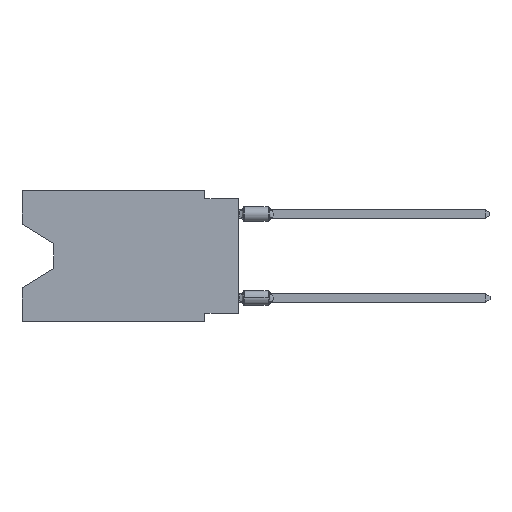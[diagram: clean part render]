
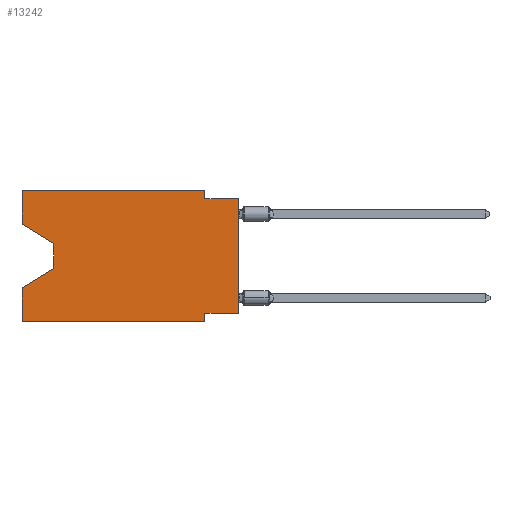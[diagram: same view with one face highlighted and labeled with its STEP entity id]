
A CAD part, left-side view. The second image highlights one B-rep face of the part: STEP entity #13242.
In plain terms, the highlighted planar face has unit normal (-1, 0, 0).
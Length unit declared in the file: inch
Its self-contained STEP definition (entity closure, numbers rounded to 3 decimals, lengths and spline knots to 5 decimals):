
#98 = DIRECTION ( 'NONE',  ( 1., 0., 0. ) ) ;
#227 = VERTEX_POINT ( 'NONE', #9976 ) ;
#761 = VERTEX_POINT ( 'NONE', #15942 ) ;
#2110 = ORIENTED_EDGE ( 'NONE', *, *, #5034, .F. ) ;
#2157 = CARTESIAN_POINT ( 'NONE',  ( 0., 0.1, -0.025 ) ) ;
#2492 = VECTOR ( 'NONE', #20686, 39.37008 ) ;
#2521 = VERTEX_POINT ( 'NONE', #2764 ) ;
#2705 = ORIENTED_EDGE ( 'NONE', *, *, #11170, .F. ) ;
#2764 = CARTESIAN_POINT ( 'NONE',  ( 0., 0., -0.025 ) ) ;
#2971 = EDGE_CURVE ( 'NONE', #761, #23270, #11813, .T. ) ;
#3758 = EDGE_CURVE ( 'NONE', #20661, #7375, #24118, .T. ) ;
#3855 = LINE ( 'NONE', #13872, #32271 ) ;
#4370 = CARTESIAN_POINT ( 'NONE',  ( 0., 0.645, -0.39 ) ) ;
#4627 = VECTOR ( 'NONE', #27420, 39.37008 ) ;
#4654 = DIRECTION ( 'NONE',  ( 0., -1., 0. ) ) ;
#5034 = EDGE_CURVE ( 'NONE', #16988, #2521, #13392, .T. ) ;
#5116 = ORIENTED_EDGE ( 'NONE', *, *, #30022, .F. ) ;
#5453 = AXIS2_PLACEMENT_3D ( 'NONE', #20775, #98, #15460 ) ;
#5732 = ORIENTED_EDGE ( 'NONE', *, *, #14408, .F. ) ;
#5986 = DIRECTION ( 'NONE',  ( 0., -1., 0. ) ) ;
#6054 = DIRECTION ( 'NONE',  ( 0., -1., 0. ) ) ;
#6690 = DIRECTION ( 'NONE',  ( 0., 0., -1. ) ) ;
#7098 = CARTESIAN_POINT ( 'NONE',  ( 0., 0.645, 0. ) ) ;
#7127 = EDGE_CURVE ( 'NONE', #15170, #16988, #24816, .T. ) ;
#7375 = VERTEX_POINT ( 'NONE', #26472 ) ;
#8446 = VECTOR ( 'NONE', #6690, 39.37008 ) ;
#9306 = CARTESIAN_POINT ( 'NONE',  ( 0., 0.1, -0.39 ) ) ;
#9571 = CARTESIAN_POINT ( 'NONE',  ( 0., 0.645, -0.10025 ) ) ;
#9764 = EDGE_CURVE ( 'NONE', #227, #2521, #15605, .T. ) ;
#9976 = CARTESIAN_POINT ( 'NONE',  ( 0., 0., -0.365 ) ) ;
#10005 = LINE ( 'NONE', #12577, #27619 ) ;
#10210 = LINE ( 'NONE', #7098, #2492 ) ;
#10726 = VECTOR ( 'NONE', #30234, 39.37008 ) ;
#11064 = CARTESIAN_POINT ( 'NONE',  ( 0., 0.645, -0.39 ) ) ;
#11170 = EDGE_CURVE ( 'NONE', #227, #29761, #3855, .T. ) ;
#11813 = LINE ( 'NONE', #9571, #15430 ) ;
#11831 = ORIENTED_EDGE ( 'NONE', *, *, #21192, .T. ) ;
#11841 = CARTESIAN_POINT ( 'NONE',  ( 0., 0.55, -0.158 ) ) ;
#12103 = EDGE_CURVE ( 'NONE', #29761, #7375, #28031, .T. ) ;
#12191 = ORIENTED_EDGE ( 'NONE', *, *, #3758, .T. ) ;
#12577 = CARTESIAN_POINT ( 'NONE',  ( 0., 0.645, 0. ) ) ;
#12833 = ORIENTED_EDGE ( 'NONE', *, *, #7127, .F. ) ;
#13202 = FACE_OUTER_BOUND ( 'NONE', #30408, .T. ) ;
#13242 = ADVANCED_FACE ( 'NONE', ( #13202 ), #28349, .F. ) ;
#13392 = LINE ( 'NONE', #29064, #26580 ) ;
#13872 = CARTESIAN_POINT ( 'NONE',  ( 0., 0., -0.365 ) ) ;
#14408 = EDGE_CURVE ( 'NONE', #26489, #15170, #10005, .T. ) ;
#14810 = DIRECTION ( 'NONE',  ( 0., 0., -1. ) ) ;
#15029 = CARTESIAN_POINT ( 'NONE',  ( 0., 0.645, 0. ) ) ;
#15170 = VERTEX_POINT ( 'NONE', #26195 ) ;
#15373 = ORIENTED_EDGE ( 'NONE', *, *, #16788, .F. ) ;
#15430 = VECTOR ( 'NONE', #27621, 39.37008 ) ;
#15460 = DIRECTION ( 'NONE',  ( 0., 0., -1. ) ) ;
#15471 = VERTEX_POINT ( 'NONE', #27386 ) ;
#15605 = LINE ( 'NONE', #23324, #16844 ) ;
#15942 = CARTESIAN_POINT ( 'NONE',  ( 0., 0.645, -0.10025 ) ) ;
#16788 = EDGE_CURVE ( 'NONE', #761, #26489, #17499, .T. ) ;
#16844 = VECTOR ( 'NONE', #18684, 39.37008 ) ;
#16988 = VERTEX_POINT ( 'NONE', #2157 ) ;
#17258 = DIRECTION ( 'NONE',  ( 0., 0., -1. ) ) ;
#17499 = LINE ( 'NONE', #24888, #10726 ) ;
#18422 = CARTESIAN_POINT ( 'NONE',  ( 0., 0.645, -0.28975 ) ) ;
#18684 = DIRECTION ( 'NONE',  ( 0., 0., 1. ) ) ;
#18733 = VECTOR ( 'NONE', #6054, 39.37008 ) ;
#19051 = VERTEX_POINT ( 'NONE', #18422 ) ;
#19495 = ORIENTED_EDGE ( 'NONE', *, *, #12103, .F. ) ;
#20333 = ORIENTED_EDGE ( 'NONE', *, *, #26400, .T. ) ;
#20661 = VERTEX_POINT ( 'NONE', #4370 ) ;
#20686 = DIRECTION ( 'NONE',  ( 0., 0., 1. ) ) ;
#20775 = CARTESIAN_POINT ( 'NONE',  ( 0., 0.645, 0. ) ) ;
#21192 = EDGE_CURVE ( 'NONE', #23270, #15471, #26508, .T. ) ;
#23270 = VERTEX_POINT ( 'NONE', #11841 ) ;
#23324 = CARTESIAN_POINT ( 'NONE',  ( 0., 0., 0. ) ) ;
#24118 = LINE ( 'NONE', #11064, #18733 ) ;
#24348 = DIRECTION ( 'NONE',  ( 0., 1., 0. ) ) ;
#24569 = ORIENTED_EDGE ( 'NONE', *, *, #9764, .T. ) ;
#24816 = LINE ( 'NONE', #27403, #27135 ) ;
#24888 = CARTESIAN_POINT ( 'NONE',  ( 0., 0.645, 0. ) ) ;
#26195 = CARTESIAN_POINT ( 'NONE',  ( 0., 0.1, 0. ) ) ;
#26400 = EDGE_CURVE ( 'NONE', #15471, #19051, #27077, .T. ) ;
#26472 = CARTESIAN_POINT ( 'NONE',  ( 0., 0.1, -0.39 ) ) ;
#26489 = VERTEX_POINT ( 'NONE', #15029 ) ;
#26508 = LINE ( 'NONE', #28585, #8446 ) ;
#26580 = VECTOR ( 'NONE', #5986, 39.37008 ) ;
#27077 = LINE ( 'NONE', #27248, #4627 ) ;
#27135 = VECTOR ( 'NONE', #17258, 39.37008 ) ;
#27248 = CARTESIAN_POINT ( 'NONE',  ( 0., 0.55, -0.232 ) ) ;
#27386 = CARTESIAN_POINT ( 'NONE',  ( 0., 0.55, -0.232 ) ) ;
#27403 = CARTESIAN_POINT ( 'NONE',  ( 0., 0.1, 0. ) ) ;
#27420 = DIRECTION ( 'NONE',  ( 0., 0.855, -0.519 ) ) ;
#27619 = VECTOR ( 'NONE', #4654, 39.37008 ) ;
#27621 = DIRECTION ( 'NONE',  ( 0., -0.855, -0.519 ) ) ;
#28031 = LINE ( 'NONE', #9306, #31232 ) ;
#28349 = PLANE ( 'NONE',  #5453 ) ;
#28585 = CARTESIAN_POINT ( 'NONE',  ( 0., 0.55, -0.158 ) ) ;
#28997 = CARTESIAN_POINT ( 'NONE',  ( 0., 0.1, -0.365 ) ) ;
#29064 = CARTESIAN_POINT ( 'NONE',  ( 0., 0., -0.025 ) ) ;
#29761 = VERTEX_POINT ( 'NONE', #28997 ) ;
#30022 = EDGE_CURVE ( 'NONE', #20661, #19051, #10210, .T. ) ;
#30234 = DIRECTION ( 'NONE',  ( 0., 0., 1. ) ) ;
#30408 = EDGE_LOOP ( 'NONE', ( #33141, #11831, #20333, #5116, #12191, #19495, #2705, #24569, #2110, #12833, #5732, #15373 ) ) ;
#31232 = VECTOR ( 'NONE', #14810, 39.37008 ) ;
#32271 = VECTOR ( 'NONE', #24348, 39.37008 ) ;
#33141 = ORIENTED_EDGE ( 'NONE', *, *, #2971, .T. ) ;
